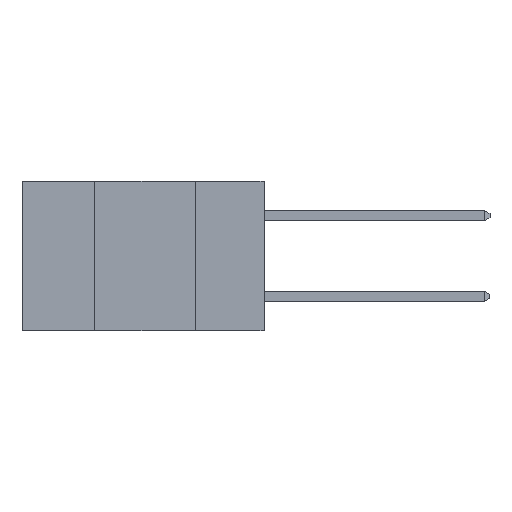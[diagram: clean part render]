
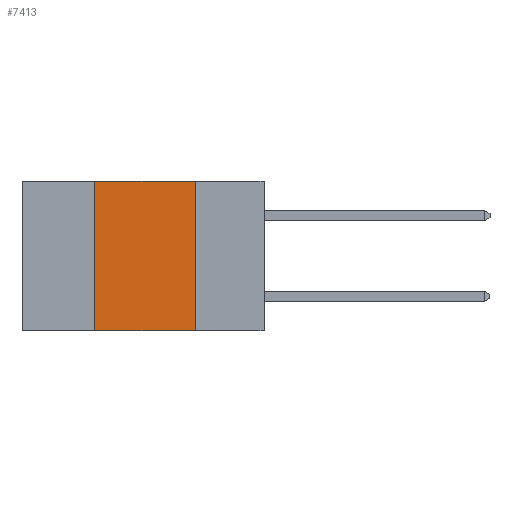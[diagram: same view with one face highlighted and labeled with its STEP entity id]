
A CAD part, left-side view. The second image highlights one B-rep face of the part: STEP entity #7413.
In plain terms, the highlighted planar face has unit normal (-1, 0, 0).
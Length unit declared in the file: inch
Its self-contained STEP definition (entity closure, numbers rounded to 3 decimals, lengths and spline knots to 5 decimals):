
#670 = EDGE_CURVE ( 'NONE', #20148, #15607, #19048, .T. ) ;
#1056 = LINE ( 'NONE', #10814, #17379 ) ;
#1976 = DIRECTION ( 'NONE',  ( 0., 0., -1. ) ) ;
#2040 = LINE ( 'NONE', #12739, #10045 ) ;
#2215 = ORIENTED_EDGE ( 'NONE', *, *, #13435, .F. ) ;
#2999 = EDGE_LOOP ( 'NONE', ( #13060, #18674, #2215, #4432 ) ) ;
#3660 = VERTEX_POINT ( 'NONE', #16214 ) ;
#4432 = ORIENTED_EDGE ( 'NONE', *, *, #8633, .T. ) ;
#4772 = LINE ( 'NONE', #10946, #12601 ) ;
#5061 = AXIS2_PLACEMENT_3D ( 'NONE', #9955, #11535, #1976 ) ;
#5323 = CARTESIAN_POINT ( 'NONE',  ( 0., 0.42, 0. ) ) ;
#6930 = CARTESIAN_POINT ( 'NONE',  ( 0., 0.17, 0. ) ) ;
#7413 = ADVANCED_FACE ( 'NONE', ( #12748 ), #8377, .F. ) ;
#7798 = EDGE_CURVE ( 'NONE', #15607, #3660, #1056, .T. ) ;
#8377 = PLANE ( 'NONE',  #5061 ) ;
#8633 = EDGE_CURVE ( 'NONE', #17504, #3660, #2040, .T. ) ;
#9955 = CARTESIAN_POINT ( 'NONE',  ( 0., 0.6, 0. ) ) ;
#10045 = VECTOR ( 'NONE', #12659, 39.37008 ) ;
#10727 = CARTESIAN_POINT ( 'NONE',  ( 0., 0.6, 0. ) ) ;
#10814 = CARTESIAN_POINT ( 'NONE',  ( 0., 0.17, 0. ) ) ;
#10834 = DIRECTION ( 'NONE',  ( 0., -1., 0. ) ) ;
#10946 = CARTESIAN_POINT ( 'NONE',  ( 0., 0.42, 0. ) ) ;
#11535 = DIRECTION ( 'NONE',  ( 1., 0., 0. ) ) ;
#12601 = VECTOR ( 'NONE', #20249, 39.37008 ) ;
#12659 = DIRECTION ( 'NONE',  ( 0., -1., 0. ) ) ;
#12739 = CARTESIAN_POINT ( 'NONE',  ( 0., 0.6, -0.37 ) ) ;
#12748 = FACE_OUTER_BOUND ( 'NONE', #2999, .T. ) ;
#13060 = ORIENTED_EDGE ( 'NONE', *, *, #7798, .F. ) ;
#13435 = EDGE_CURVE ( 'NONE', #17504, #20148, #4772, .T. ) ;
#14898 = VECTOR ( 'NONE', #10834, 39.37008 ) ;
#15607 = VERTEX_POINT ( 'NONE', #6930 ) ;
#16214 = CARTESIAN_POINT ( 'NONE',  ( 0., 0.17, -0.37 ) ) ;
#17077 = DIRECTION ( 'NONE',  ( 0., 0., -1. ) ) ;
#17379 = VECTOR ( 'NONE', #17077, 39.37008 ) ;
#17504 = VERTEX_POINT ( 'NONE', #17583 ) ;
#17583 = CARTESIAN_POINT ( 'NONE',  ( 0., 0.42, -0.37 ) ) ;
#18674 = ORIENTED_EDGE ( 'NONE', *, *, #670, .F. ) ;
#19048 = LINE ( 'NONE', #10727, #14898 ) ;
#20148 = VERTEX_POINT ( 'NONE', #5323 ) ;
#20249 = DIRECTION ( 'NONE',  ( 0., 0., 1. ) ) ;
